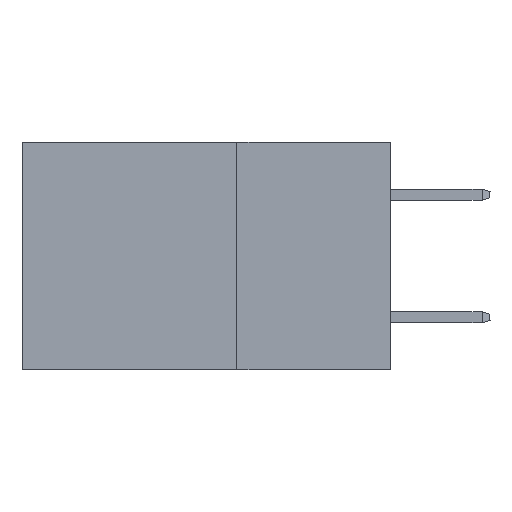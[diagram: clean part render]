
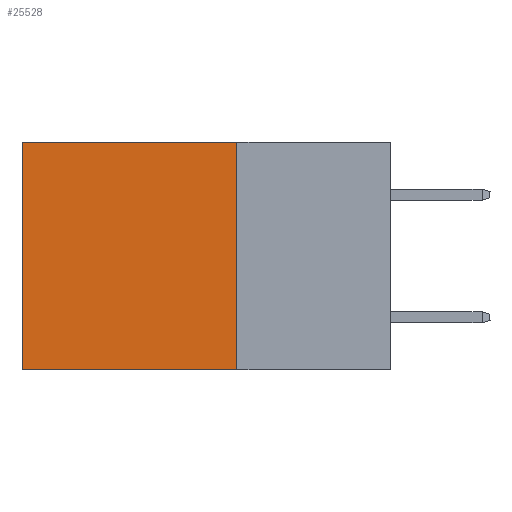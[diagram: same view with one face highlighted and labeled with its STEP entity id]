
A CAD part, left-side view. The second image highlights one B-rep face of the part: STEP entity #25528.
In plain terms, the highlighted planar face has unit normal (-1, 0, 0).
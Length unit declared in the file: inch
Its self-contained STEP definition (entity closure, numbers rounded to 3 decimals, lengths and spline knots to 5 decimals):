
#571 = EDGE_LOOP ( 'NONE', ( #36148, #17900, #8516, #45631 ) ) ;
#695 = AXIS2_PLACEMENT_3D ( 'NONE', #27064, #30291, #41291 ) ;
#704 = EDGE_CURVE ( 'NONE', #42711, #2661, #7558, .T. ) ;
#2661 = VERTEX_POINT ( 'NONE', #28859 ) ;
#4145 = DIRECTION ( 'NONE',  ( 0., 0., -1. ) ) ;
#4387 = VECTOR ( 'NONE', #4145, 39.37008 ) ;
#4823 = VERTEX_POINT ( 'NONE', #5270 ) ;
#5270 = CARTESIAN_POINT ( 'NONE',  ( 0.2875, 0.25, 0. ) ) ;
#5397 = LINE ( 'NONE', #5704, #33690 ) ;
#5704 = CARTESIAN_POINT ( 'NONE',  ( 0.2875, 0.6, 0. ) ) ;
#6017 = DIRECTION ( 'NONE',  ( 0., 0., -1. ) ) ;
#6406 = DIRECTION ( 'NONE',  ( 0., 1., 0. ) ) ;
#7558 = LINE ( 'NONE', #7778, #16414 ) ;
#7778 = CARTESIAN_POINT ( 'NONE',  ( 0.2875, 0.25, -0.37 ) ) ;
#8516 = ORIENTED_EDGE ( 'NONE', *, *, #11638, .F. ) ;
#9217 = PLANE ( 'NONE',  #695 ) ;
#9700 = CARTESIAN_POINT ( 'NONE',  ( 0.2875, 0.25, 0. ) ) ;
#11638 = EDGE_CURVE ( 'NONE', #4823, #42711, #20469, .T. ) ;
#12759 = CARTESIAN_POINT ( 'NONE',  ( 0.2875, 0.6, 0. ) ) ;
#13762 = FACE_OUTER_BOUND ( 'NONE', #571, .T. ) ;
#14201 = VECTOR ( 'NONE', #6406, 39.37008 ) ;
#16414 = VECTOR ( 'NONE', #18953, 39.37008 ) ;
#16447 = EDGE_CURVE ( 'NONE', #33454, #2661, #5397, .T. ) ;
#17900 = ORIENTED_EDGE ( 'NONE', *, *, #704, .F. ) ;
#18953 = DIRECTION ( 'NONE',  ( 0., 1., 0. ) ) ;
#20469 = LINE ( 'NONE', #22173, #4387 ) ;
#22173 = CARTESIAN_POINT ( 'NONE',  ( 0.2875, 0.25, 0. ) ) ;
#25528 = ADVANCED_FACE ( 'NONE', ( #13762 ), #9217, .F. ) ;
#27064 = CARTESIAN_POINT ( 'NONE',  ( 0.2875, 0.25, 0. ) ) ;
#28859 = CARTESIAN_POINT ( 'NONE',  ( 0.2875, 0.6, -0.37 ) ) ;
#30291 = DIRECTION ( 'NONE',  ( 1., 0., 0. ) ) ;
#31958 = LINE ( 'NONE', #9700, #14201 ) ;
#33454 = VERTEX_POINT ( 'NONE', #12759 ) ;
#33690 = VECTOR ( 'NONE', #6017, 39.37008 ) ;
#36148 = ORIENTED_EDGE ( 'NONE', *, *, #16447, .T. ) ;
#41222 = EDGE_CURVE ( 'NONE', #4823, #33454, #31958, .T. ) ;
#41291 = DIRECTION ( 'NONE',  ( 0., 0., -1. ) ) ;
#42711 = VERTEX_POINT ( 'NONE', #45042 ) ;
#45042 = CARTESIAN_POINT ( 'NONE',  ( 0.2875, 0.25, -0.37 ) ) ;
#45631 = ORIENTED_EDGE ( 'NONE', *, *, #41222, .T. ) ;
